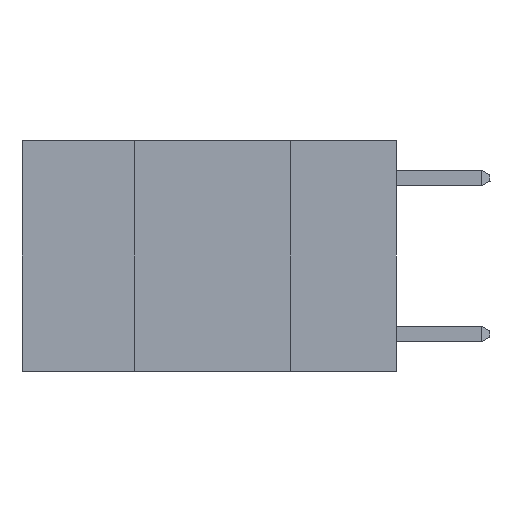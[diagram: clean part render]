
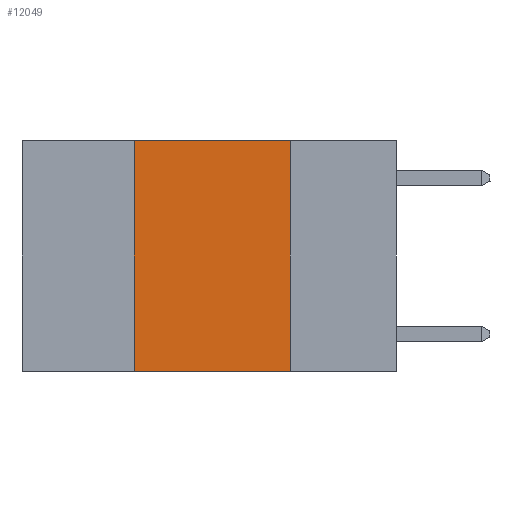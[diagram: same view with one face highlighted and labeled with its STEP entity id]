
A CAD part, left-side view. The second image highlights one B-rep face of the part: STEP entity #12049.
In plain terms, the highlighted planar face has unit normal (-1, 0, 0).
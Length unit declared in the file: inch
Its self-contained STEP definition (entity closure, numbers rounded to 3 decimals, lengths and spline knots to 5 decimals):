
#354 = DIRECTION ( 'NONE',  ( 1., 0., 0. ) ) ;
#2030 = VECTOR ( 'NONE', #2395, 39.37008 ) ;
#2395 = DIRECTION ( 'NONE',  ( 0., -1., 0. ) ) ;
#2436 = EDGE_CURVE ( 'NONE', #18020, #2639, #6493, .T. ) ;
#2639 = VERTEX_POINT ( 'NONE', #10788 ) ;
#2720 = VERTEX_POINT ( 'NONE', #3650 ) ;
#3650 = CARTESIAN_POINT ( 'NONE',  ( 0., 0.17, -0.37 ) ) ;
#4734 = DIRECTION ( 'NONE',  ( 0., -1., 0. ) ) ;
#5906 = LINE ( 'NONE', #15134, #2030 ) ;
#6493 = LINE ( 'NONE', #16003, #17169 ) ;
#6568 = CARTESIAN_POINT ( 'NONE',  ( 0., 0.17, 0. ) ) ;
#7289 = LINE ( 'NONE', #6568, #11037 ) ;
#7449 = FACE_OUTER_BOUND ( 'NONE', #8200, .T. ) ;
#8200 = EDGE_LOOP ( 'NONE', ( #9352, #11886, #11115, #12271 ) ) ;
#9045 = PLANE ( 'NONE',  #11771 ) ;
#9320 = LINE ( 'NONE', #18055, #10167 ) ;
#9352 = ORIENTED_EDGE ( 'NONE', *, *, #16365, .F. ) ;
#10167 = VECTOR ( 'NONE', #11237, 39.37008 ) ;
#10437 = DIRECTION ( 'NONE',  ( 0., 0., -1. ) ) ;
#10788 = CARTESIAN_POINT ( 'NONE',  ( 0., 0.17, 0. ) ) ;
#11037 = VECTOR ( 'NONE', #12212, 39.37008 ) ;
#11115 = ORIENTED_EDGE ( 'NONE', *, *, #16946, .F. ) ;
#11237 = DIRECTION ( 'NONE',  ( 0., 0., 1. ) ) ;
#11771 = AXIS2_PLACEMENT_3D ( 'NONE', #17299, #354, #10437 ) ;
#11886 = ORIENTED_EDGE ( 'NONE', *, *, #2436, .F. ) ;
#12049 = ADVANCED_FACE ( 'NONE', ( #7449 ), #9045, .F. ) ;
#12212 = DIRECTION ( 'NONE',  ( 0., 0., -1. ) ) ;
#12271 = ORIENTED_EDGE ( 'NONE', *, *, #17706, .T. ) ;
#15134 = CARTESIAN_POINT ( 'NONE',  ( 0., 0.6, -0.37 ) ) ;
#15658 = CARTESIAN_POINT ( 'NONE',  ( 0., 0.42, 0. ) ) ;
#15863 = VERTEX_POINT ( 'NONE', #18187 ) ;
#16003 = CARTESIAN_POINT ( 'NONE',  ( 0., 0.6, 0. ) ) ;
#16365 = EDGE_CURVE ( 'NONE', #2639, #2720, #7289, .T. ) ;
#16946 = EDGE_CURVE ( 'NONE', #15863, #18020, #9320, .T. ) ;
#17169 = VECTOR ( 'NONE', #4734, 39.37008 ) ;
#17299 = CARTESIAN_POINT ( 'NONE',  ( 0., 0.6, 0. ) ) ;
#17706 = EDGE_CURVE ( 'NONE', #15863, #2720, #5906, .T. ) ;
#18020 = VERTEX_POINT ( 'NONE', #15658 ) ;
#18055 = CARTESIAN_POINT ( 'NONE',  ( 0., 0.42, 0. ) ) ;
#18187 = CARTESIAN_POINT ( 'NONE',  ( 0., 0.42, -0.37 ) ) ;
